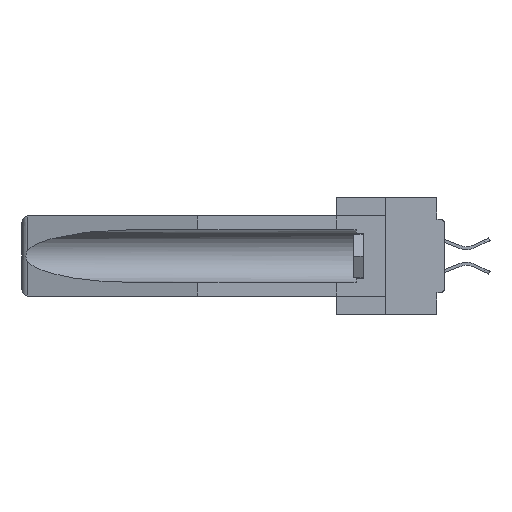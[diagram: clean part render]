
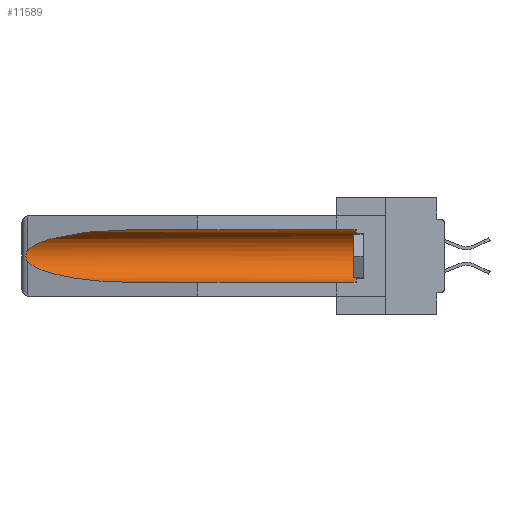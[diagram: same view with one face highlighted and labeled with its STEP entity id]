
A CAD part, left-side view. The second image highlights one B-rep face of the part: STEP entity #11589.
In plain terms, the highlighted cylindrical face has radius 2.857 mm (diameter 5.715 mm), a partial arc.
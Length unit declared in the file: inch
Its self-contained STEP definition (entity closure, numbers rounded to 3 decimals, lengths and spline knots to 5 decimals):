
#528 = DIRECTION ( 'NONE',  ( 0., 0., 1. ) ) ;
#1223 = CARTESIAN_POINT ( 'NONE',  ( 0.155, 1.07973, -0.059 ) ) ;
#1533 = LINE ( 'NONE', #23975, #18539 ) ;
#1564 = CARTESIAN_POINT ( 'NONE',  ( 0.2675, 1.53308, -0.16763 ) ) ;
#2170 = ORIENTED_EDGE ( 'NONE', *, *, #23965, .T. ) ;
#4635 = CARTESIAN_POINT ( 'NONE',  ( 0.155, 0.126, -0.059 ) ) ;
#4651 = DIRECTION ( 'NONE',  ( 0., 1., 0. ) ) ;
#4901 = CARTESIAN_POINT ( 'NONE',  ( 0.2673, 1.5327, -0.16383 ) ) ;
#5806 = ORIENTED_EDGE ( 'NONE', *, *, #37573, .T. ) ;
#6770 = EDGE_CURVE ( 'NONE', #15986, #31212, #19494, .T. ) ;
#7064 = DIRECTION ( 'NONE',  ( 0., -1., 0. ) ) ;
#7382 = ORIENTED_EDGE ( 'NONE', *, *, #6770, .F. ) ;
#8551 = CARTESIAN_POINT ( 'NONE',  ( 0.155, -0.30754, -0.1715 ) ) ;
#9912 = FACE_OUTER_BOUND ( 'NONE', #12209, .T. ) ;
#10338 = CARTESIAN_POINT ( 'NONE',  ( 0.21114, 1.30732, -0.284 ) ) ;
#10390 = AXIS2_PLACEMENT_3D ( 'NONE', #26272, #7064, #528 ) ;
#10592 =( BOUNDED_CURVE ( )  B_SPLINE_CURVE ( 3, ( #31497, #31360, #41115, #21713 ),
 .UNSPECIFIED., .F., .T. ) 
 B_SPLINE_CURVE_WITH_KNOTS ( ( 4, 4 ),
 ( 4.71239, 6.08839 ),
 .UNSPECIFIED. ) 
 CURVE ( )  GEOMETRIC_REPRESENTATION_ITEM ( )  RATIONAL_B_SPLINE_CURVE ( ( 1., 0.848, 0.848, 1. ) ) 
 REPRESENTATION_ITEM ( '' )  );
#11006 = VERTEX_POINT ( 'NONE', #34006 ) ;
#11042 = CARTESIAN_POINT ( 'NONE',  ( 0.2673, 1.53269, -0.17917 ) ) ;
#11067 = ORIENTED_EDGE ( 'NONE', *, *, #14769, .T. ) ;
#11589 = ADVANCED_FACE ( 'NONE', ( #9912 ), #22893, .F. ) ;
#12209 = EDGE_LOOP ( 'NONE', ( #34243, #5806, #2170, #7382, #18544, #11067 ) ) ;
#12664 = EDGE_CURVE ( 'NONE', #15986, #35405, #23829, .T. ) ;
#13113 = CARTESIAN_POINT ( 'NONE',  ( 0.155, 1.07973, -0.284 ) ) ;
#13584 = CARTESIAN_POINT ( 'NONE',  ( 0.155, 0.126, -0.284 ) ) ;
#13637 = B_SPLINE_CURVE_WITH_KNOTS ( 'NONE', 3,
 ( #19888, #33172, #13964, #4901, #1564, #23959, #11042, #33578, #30789, #27593 ),
 .UNSPECIFIED., .F., .F.,
 ( 4, 2, 2, 2, 4 ),
 ( 0., 0.00029, 0.00058, 0.00087, 0.00117 ),
 .UNSPECIFIED. ) ;
#13964 = CARTESIAN_POINT ( 'NONE',  ( 0.26654, 1.53092, -0.15636 ) ) ;
#14769 = EDGE_CURVE ( 'NONE', #35405, #27903, #1533, .T. ) ;
#15678 = CARTESIAN_POINT ( 'NONE',  ( 0.26537, 1.52718, -0.19328 ) ) ;
#15986 = VERTEX_POINT ( 'NONE', #13584 ) ;
#18539 = VECTOR ( 'NONE', #4651, 39.37008 ) ;
#18544 = ORIENTED_EDGE ( 'NONE', *, *, #12664, .T. ) ;
#18909 = CARTESIAN_POINT ( 'NONE',  ( 0.26537, 1.52718, -0.14972 ) ) ;
#19494 = LINE ( 'NONE', #29596, #34499 ) ;
#19888 = CARTESIAN_POINT ( 'NONE',  ( 0.26537, 1.52718, -0.14972 ) ) ;
#21713 = CARTESIAN_POINT ( 'NONE',  ( 0.26537, 1.52718, -0.14972 ) ) ;
#22893 = CYLINDRICAL_SURFACE ( 'NONE', #41220, 0.1125 ) ;
#23829 = CIRCLE ( 'NONE', #10390, 0.1125 ) ;
#23959 = CARTESIAN_POINT ( 'NONE',  ( 0.2675, 1.53308, -0.17534 ) ) ;
#23965 = EDGE_CURVE ( 'NONE', #11006, #31212, #38835, .T. ) ;
#23975 = CARTESIAN_POINT ( 'NONE',  ( 0.155, -0.30754, -0.059 ) ) ;
#24838 = DIRECTION ( 'NONE',  ( 0., 1., 0. ) ) ;
#26272 = CARTESIAN_POINT ( 'NONE',  ( 0.155, 0.126, -0.1715 ) ) ;
#26562 = DIRECTION ( 'NONE',  ( 0., 1., 0. ) ) ;
#26664 = EDGE_CURVE ( 'NONE', #27903, #40803, #10592, .T. ) ;
#27593 = CARTESIAN_POINT ( 'NONE',  ( 0.26537, 1.52718, -0.19328 ) ) ;
#27903 = VERTEX_POINT ( 'NONE', #1223 ) ;
#29596 = CARTESIAN_POINT ( 'NONE',  ( 0.155, -0.30754, -0.284 ) ) ;
#29671 = CARTESIAN_POINT ( 'NONE',  ( 0.25451, 1.48313, -0.24835 ) ) ;
#30789 = CARTESIAN_POINT ( 'NONE',  ( 0.26597, 1.5296, -0.19026 ) ) ;
#31110 = DIRECTION ( 'NONE',  ( 0., 0., 1. ) ) ;
#31212 = VERTEX_POINT ( 'NONE', #13113 ) ;
#31360 = CARTESIAN_POINT ( 'NONE',  ( 0.21114, 1.30732, -0.059 ) ) ;
#31497 = CARTESIAN_POINT ( 'NONE',  ( 0.155, 1.07973, -0.059 ) ) ;
#33172 = CARTESIAN_POINT ( 'NONE',  ( 0.26597, 1.52961, -0.15275 ) ) ;
#33578 = CARTESIAN_POINT ( 'NONE',  ( 0.26655, 1.53094, -0.18657 ) ) ;
#34006 = CARTESIAN_POINT ( 'NONE',  ( 0.26537, 1.52718, -0.19328 ) ) ;
#34243 = ORIENTED_EDGE ( 'NONE', *, *, #26664, .T. ) ;
#34499 = VECTOR ( 'NONE', #26562, 39.37008 ) ;
#35405 = VERTEX_POINT ( 'NONE', #4635 ) ;
#35841 = CARTESIAN_POINT ( 'NONE',  ( 0.155, 1.07973, -0.284 ) ) ;
#37573 = EDGE_CURVE ( 'NONE', #40803, #11006, #13637, .T. ) ;
#38835 =( BOUNDED_CURVE ( )  B_SPLINE_CURVE ( 3, ( #15678, #29671, #10338, #35841 ),
 .UNSPECIFIED., .F., .T. ) 
 B_SPLINE_CURVE_WITH_KNOTS ( ( 4, 4 ),
 ( 0.1948, 1.5708 ),
 .UNSPECIFIED. ) 
 CURVE ( )  GEOMETRIC_REPRESENTATION_ITEM ( )  RATIONAL_B_SPLINE_CURVE ( ( 1., 0.848, 0.848, 1. ) ) 
 REPRESENTATION_ITEM ( '' )  );
#40803 = VERTEX_POINT ( 'NONE', #18909 ) ;
#41115 = CARTESIAN_POINT ( 'NONE',  ( 0.25451, 1.48313, -0.09465 ) ) ;
#41220 = AXIS2_PLACEMENT_3D ( 'NONE', #8551, #24838, #31110 ) ;
